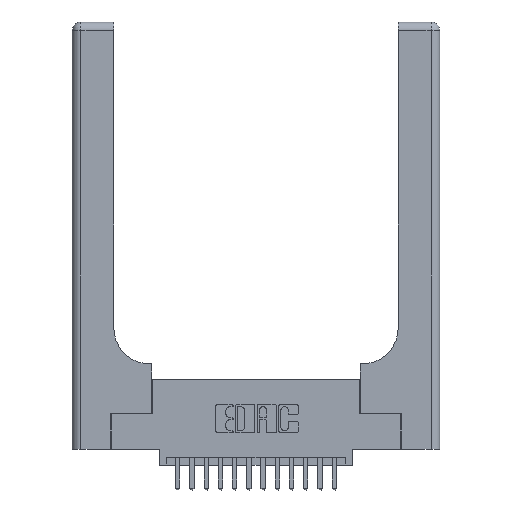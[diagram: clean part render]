
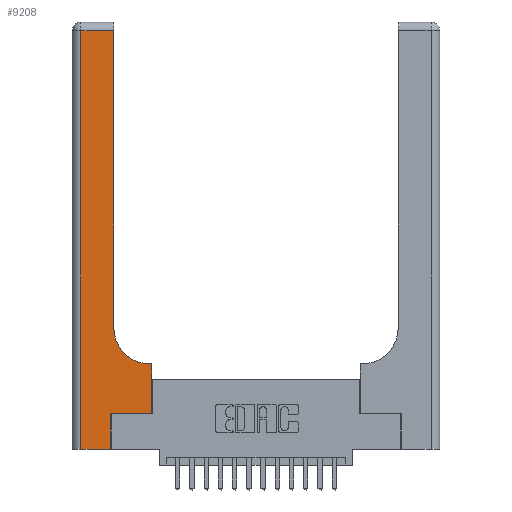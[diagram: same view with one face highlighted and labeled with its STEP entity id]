
A CAD part, top view. The second image highlights one B-rep face of the part: STEP entity #9208.
In plain terms, the highlighted planar face has unit normal (0, 0, 1).
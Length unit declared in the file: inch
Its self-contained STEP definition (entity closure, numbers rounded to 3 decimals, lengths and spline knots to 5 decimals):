
#50 = CARTESIAN_POINT ( 'NONE',  ( 0.2915, 2.94, 0.37 ) ) ;
#565 = CARTESIAN_POINT ( 'NONE',  ( 0., 3., 0.37 ) ) ;
#820 = VECTOR ( 'NONE', #16241, 39.37008 ) ;
#900 = EDGE_CURVE ( 'NONE', #18552, #1351, #4821, .T. ) ;
#1351 = VERTEX_POINT ( 'NONE', #2721 ) ;
#1481 = EDGE_LOOP ( 'NONE', ( #10574, #9421, #5743, #8540, #12947, #4907, #14557, #13222, #1941 ) ) ;
#1816 = CARTESIAN_POINT ( 'NONE',  ( 0.269, 0.25, 0.37 ) ) ;
#1941 = ORIENTED_EDGE ( 'NONE', *, *, #11590, .T. ) ;
#2056 = CARTESIAN_POINT ( 'NONE',  ( 0., 2.94, 0.37 ) ) ;
#2449 = VERTEX_POINT ( 'NONE', #50 ) ;
#2632 = AXIS2_PLACEMENT_3D ( 'NONE', #13732, #5031, #15152 ) ;
#2721 = CARTESIAN_POINT ( 'NONE',  ( 0.06, 0., 0.37 ) ) ;
#3255 = CARTESIAN_POINT ( 'NONE',  ( 0.06, 2.94, 0.37 ) ) ;
#3448 = LINE ( 'NONE', #2056, #10712 ) ;
#3600 = DIRECTION ( 'NONE',  ( 0., 0., -1. ) ) ;
#3672 = EDGE_CURVE ( 'NONE', #6510, #10974, #9544, .T. ) ;
#4552 = VECTOR ( 'NONE', #5899, 39.37008 ) ;
#4821 = LINE ( 'NONE', #17933, #820 ) ;
#4907 = ORIENTED_EDGE ( 'NONE', *, *, #6426, .T. ) ;
#5031 = DIRECTION ( 'NONE',  ( 0., 0., -1. ) ) ;
#5043 = DIRECTION ( 'NONE',  ( -1., 0., 0. ) ) ;
#5417 = VERTEX_POINT ( 'NONE', #10598 ) ;
#5743 = ORIENTED_EDGE ( 'NONE', *, *, #900, .T. ) ;
#5899 = DIRECTION ( 'NONE',  ( 1., 0., 0. ) ) ;
#6195 = VECTOR ( 'NONE', #9553, 39.37008 ) ;
#6245 = VERTEX_POINT ( 'NONE', #11574 ) ;
#6426 = EDGE_CURVE ( 'NONE', #16960, #6245, #11260, .T. ) ;
#6510 = VERTEX_POINT ( 'NONE', #12227 ) ;
#6709 = EDGE_CURVE ( 'NONE', #14289, #2449, #10581, .T. ) ;
#7123 = VECTOR ( 'NONE', #7454, 39.37008 ) ;
#7454 = DIRECTION ( 'NONE',  ( 0., 1., 0. ) ) ;
#8221 = LINE ( 'NONE', #10868, #12128 ) ;
#8300 = VECTOR ( 'NONE', #10554, 39.37008 ) ;
#8540 = ORIENTED_EDGE ( 'NONE', *, *, #18425, .T. ) ;
#9208 = ADVANCED_FACE ( 'NONE', ( #15107 ), #12304, .F. ) ;
#9421 = ORIENTED_EDGE ( 'NONE', *, *, #11196, .T. ) ;
#9544 = LINE ( 'NONE', #15346, #6195 ) ;
#9553 = DIRECTION ( 'NONE',  ( -1., 0., 0. ) ) ;
#10554 = DIRECTION ( 'NONE',  ( 1., 0., 0. ) ) ;
#10574 = ORIENTED_EDGE ( 'NONE', *, *, #6709, .T. ) ;
#10581 = LINE ( 'NONE', #16935, #14452 ) ;
#10598 = CARTESIAN_POINT ( 'NONE',  ( 0.269, 0., 0.37 ) ) ;
#10712 = VECTOR ( 'NONE', #5043, 39.37008 ) ;
#10868 = CARTESIAN_POINT ( 'NONE',  ( 0.269, 0., 0.37 ) ) ;
#10974 = VERTEX_POINT ( 'NONE', #11812 ) ;
#11196 = EDGE_CURVE ( 'NONE', #2449, #18552, #3448, .T. ) ;
#11260 = LINE ( 'NONE', #1816, #8300 ) ;
#11502 = CARTESIAN_POINT ( 'NONE',  ( 0.2915, 0.85, 0.37 ) ) ;
#11574 = CARTESIAN_POINT ( 'NONE',  ( 0.5585, 0.25, 0.37 ) ) ;
#11590 = EDGE_CURVE ( 'NONE', #10974, #14289, #15455, .T. ) ;
#11812 = CARTESIAN_POINT ( 'NONE',  ( 0.5415, 0.6, 0.37 ) ) ;
#12128 = VECTOR ( 'NONE', #16636, 39.37008 ) ;
#12227 = CARTESIAN_POINT ( 'NONE',  ( 0.5585, 0.6, 0.37 ) ) ;
#12304 = PLANE ( 'NONE',  #17274 ) ;
#12947 = ORIENTED_EDGE ( 'NONE', *, *, #16866, .T. ) ;
#13222 = ORIENTED_EDGE ( 'NONE', *, *, #3672, .T. ) ;
#13732 = CARTESIAN_POINT ( 'NONE',  ( 0.5415, 0.85, 0.37 ) ) ;
#13783 = DIRECTION ( 'NONE',  ( -1., 0., 0. ) ) ;
#14058 = DIRECTION ( 'NONE',  ( 0., 1., 0. ) ) ;
#14289 = VERTEX_POINT ( 'NONE', #11502 ) ;
#14452 = VECTOR ( 'NONE', #14058, 39.37008 ) ;
#14557 = ORIENTED_EDGE ( 'NONE', *, *, #16669, .T. ) ;
#14695 = CARTESIAN_POINT ( 'NONE',  ( 0.5585, 0.25, 0.37 ) ) ;
#15107 = FACE_OUTER_BOUND ( 'NONE', #1481, .T. ) ;
#15152 = DIRECTION ( 'NONE',  ( 1., 0., 0. ) ) ;
#15346 = CARTESIAN_POINT ( 'NONE',  ( 0.2915, 0.6, 0.37 ) ) ;
#15429 = CARTESIAN_POINT ( 'NONE',  ( 0.269, 0.25, 0.37 ) ) ;
#15455 = CIRCLE ( 'NONE', #2632, 0.25 ) ;
#16129 = LINE ( 'NONE', #17447, #4552 ) ;
#16241 = DIRECTION ( 'NONE',  ( 0., -1., 0. ) ) ;
#16636 = DIRECTION ( 'NONE',  ( 0., 1., 0. ) ) ;
#16669 = EDGE_CURVE ( 'NONE', #6245, #6510, #18626, .T. ) ;
#16866 = EDGE_CURVE ( 'NONE', #5417, #16960, #8221, .T. ) ;
#16935 = CARTESIAN_POINT ( 'NONE',  ( 0.2915, 3., 0.37 ) ) ;
#16960 = VERTEX_POINT ( 'NONE', #15429 ) ;
#17274 = AXIS2_PLACEMENT_3D ( 'NONE', #565, #3600, #13783 ) ;
#17447 = CARTESIAN_POINT ( 'NONE',  ( 0., 0., 0.37 ) ) ;
#17933 = CARTESIAN_POINT ( 'NONE',  ( 0.06, 3., 0.37 ) ) ;
#18425 = EDGE_CURVE ( 'NONE', #1351, #5417, #16129, .T. ) ;
#18552 = VERTEX_POINT ( 'NONE', #3255 ) ;
#18626 = LINE ( 'NONE', #14695, #7123 ) ;
